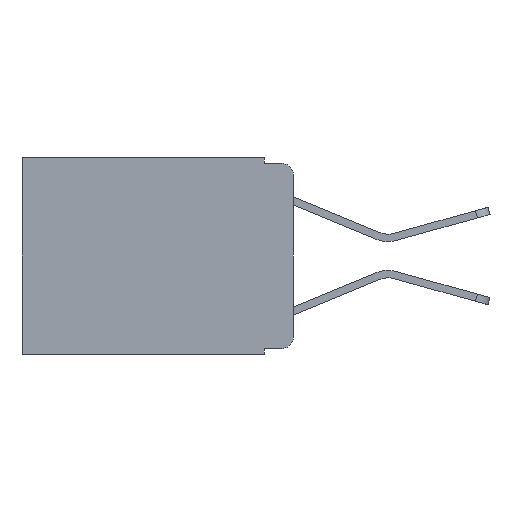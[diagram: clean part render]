
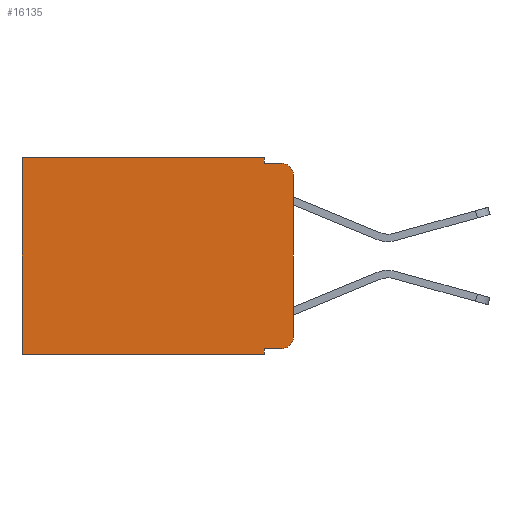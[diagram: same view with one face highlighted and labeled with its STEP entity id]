
A CAD part, left-side view. The second image highlights one B-rep face of the part: STEP entity #16135.
In plain terms, the highlighted planar face has unit normal (-1, 0, 0).
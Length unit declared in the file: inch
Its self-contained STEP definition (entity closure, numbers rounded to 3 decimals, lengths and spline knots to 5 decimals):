
#930 = DIRECTION ( 'NONE',  ( 0., 0., -1. ) ) ;
#975 = AXIS2_PLACEMENT_3D ( 'NONE', #14373, #9306, #9220 ) ;
#996 = EDGE_CURVE ( 'NONE', #8106, #8178, #16025, .T. ) ;
#1023 = CIRCLE ( 'NONE', #5226, 0.02 ) ;
#1413 = DIRECTION ( 'NONE',  ( 0., -1., 0. ) ) ;
#1445 = DIRECTION ( 'NONE',  ( 0., 0., -1. ) ) ;
#1476 = EDGE_CURVE ( 'NONE', #8192, #5066, #4135, .T. ) ;
#1765 = FACE_OUTER_BOUND ( 'NONE', #11702, .T. ) ;
#2794 = CARTESIAN_POINT ( 'NONE',  ( 0.298, 0.473, 0. ) ) ;
#2833 = AXIS2_PLACEMENT_3D ( 'NONE', #5784, #11110, #16434 ) ;
#2936 = ORIENTED_EDGE ( 'NONE', *, *, #5805, .F. ) ;
#3048 = CARTESIAN_POINT ( 'NONE',  ( 0.298, 0.051, -0.333 ) ) ;
#3153 = DIRECTION ( 'NONE',  ( -1., 0., 0. ) ) ;
#3159 = EDGE_CURVE ( 'NONE', #16995, #5421, #5808, .T. ) ;
#3177 = ORIENTED_EDGE ( 'NONE', *, *, #3159, .F. ) ;
#3296 = CARTESIAN_POINT ( 'NONE',  ( 0.298, 0., -0.313 ) ) ;
#3312 = LINE ( 'NONE', #7144, #11149 ) ;
#3498 = EDGE_CURVE ( 'NONE', #16995, #8106, #12305, .T. ) ;
#4135 = LINE ( 'NONE', #5103, #10213 ) ;
#4158 = CARTESIAN_POINT ( 'NONE',  ( 0.298, 0.473, 0. ) ) ;
#4216 = DIRECTION ( 'NONE',  ( 0., 0., -1. ) ) ;
#4322 = LINE ( 'NONE', #5625, #15662 ) ;
#4462 = CARTESIAN_POINT ( 'NONE',  ( 0.298, 0.02, -0.333 ) ) ;
#4895 = LINE ( 'NONE', #14287, #6115 ) ;
#5066 = VERTEX_POINT ( 'NONE', #14925 ) ;
#5103 = CARTESIAN_POINT ( 'NONE',  ( 0.298, 0.051, -0.01 ) ) ;
#5226 = AXIS2_PLACEMENT_3D ( 'NONE', #12319, #3153, #4216 ) ;
#5421 = VERTEX_POINT ( 'NONE', #7190 ) ;
#5423 = VERTEX_POINT ( 'NONE', #8684 ) ;
#5426 = CARTESIAN_POINT ( 'NONE',  ( 0.298, 0.051, -0.333 ) ) ;
#5625 = CARTESIAN_POINT ( 'NONE',  ( 0.298, 0., 0. ) ) ;
#5691 = LINE ( 'NONE', #11283, #7741 ) ;
#5784 = CARTESIAN_POINT ( 'NONE',  ( 0.298, 0., 0. ) ) ;
#5805 = EDGE_CURVE ( 'NONE', #5423, #8178, #4322, .T. ) ;
#5808 = LINE ( 'NONE', #7441, #16884 ) ;
#6003 = CARTESIAN_POINT ( 'NONE',  ( 0.298, 0.051, 0. ) ) ;
#6020 = ORIENTED_EDGE ( 'NONE', *, *, #8241, .T. ) ;
#6115 = VECTOR ( 'NONE', #930, 39.37008 ) ;
#6251 = EDGE_CURVE ( 'NONE', #5421, #10472, #3312, .T. ) ;
#6329 = EDGE_CURVE ( 'NONE', #16472, #9595, #5691, .T. ) ;
#6576 = VECTOR ( 'NONE', #1445, 39.37008 ) ;
#6862 = EDGE_CURVE ( 'NONE', #16472, #8192, #4895, .T. ) ;
#6928 = LINE ( 'NONE', #4158, #6576 ) ;
#7073 = PLANE ( 'NONE',  #2833 ) ;
#7144 = CARTESIAN_POINT ( 'NONE',  ( 0.298, 0., -0.343 ) ) ;
#7190 = CARTESIAN_POINT ( 'NONE',  ( 0.298, 0.051, -0.343 ) ) ;
#7256 = CARTESIAN_POINT ( 'NONE',  ( 0.298, 0.473, -0.343 ) ) ;
#7322 = ORIENTED_EDGE ( 'NONE', *, *, #1476, .F. ) ;
#7339 = ORIENTED_EDGE ( 'NONE', *, *, #996, .T. ) ;
#7441 = CARTESIAN_POINT ( 'NONE',  ( 0.298, 0.051, 0. ) ) ;
#7741 = VECTOR ( 'NONE', #9791, 39.37008 ) ;
#7961 = ORIENTED_EDGE ( 'NONE', *, *, #6862, .F. ) ;
#8087 = ORIENTED_EDGE ( 'NONE', *, *, #3498, .T. ) ;
#8106 = VERTEX_POINT ( 'NONE', #4462 ) ;
#8178 = VERTEX_POINT ( 'NONE', #3296 ) ;
#8192 = VERTEX_POINT ( 'NONE', #16401 ) ;
#8241 = EDGE_CURVE ( 'NONE', #9595, #10472, #6928, .T. ) ;
#8551 = ORIENTED_EDGE ( 'NONE', *, *, #12095, .T. ) ;
#8684 = CARTESIAN_POINT ( 'NONE',  ( 0.298, 0., -0.03 ) ) ;
#9220 = DIRECTION ( 'NONE',  ( 0., 0., -1. ) ) ;
#9306 = DIRECTION ( 'NONE',  ( -1., 0., 0. ) ) ;
#9310 = VECTOR ( 'NONE', #9506, 39.37008 ) ;
#9506 = DIRECTION ( 'NONE',  ( 0., -1., 0. ) ) ;
#9595 = VERTEX_POINT ( 'NONE', #2794 ) ;
#9791 = DIRECTION ( 'NONE',  ( 0., 1., 0. ) ) ;
#10213 = VECTOR ( 'NONE', #1413, 39.37008 ) ;
#10472 = VERTEX_POINT ( 'NONE', #7256 ) ;
#11110 = DIRECTION ( 'NONE',  ( 1., 0., 0. ) ) ;
#11149 = VECTOR ( 'NONE', #15015, 39.37008 ) ;
#11283 = CARTESIAN_POINT ( 'NONE',  ( 0.298, 0., 0. ) ) ;
#11702 = EDGE_LOOP ( 'NONE', ( #2936, #8551, #7322, #7961, #17272, #6020, #15754, #3177, #8087, #7339 ) ) ;
#12095 = EDGE_CURVE ( 'NONE', #5423, #5066, #1023, .T. ) ;
#12305 = LINE ( 'NONE', #3048, #9310 ) ;
#12319 = CARTESIAN_POINT ( 'NONE',  ( 0.298, 0.02, -0.03 ) ) ;
#13301 = DIRECTION ( 'NONE',  ( 0., 0., -1. ) ) ;
#14287 = CARTESIAN_POINT ( 'NONE',  ( 0.298, 0.051, 0. ) ) ;
#14373 = CARTESIAN_POINT ( 'NONE',  ( 0.298, 0.02, -0.313 ) ) ;
#14925 = CARTESIAN_POINT ( 'NONE',  ( 0.298, 0.02, -0.01 ) ) ;
#15015 = DIRECTION ( 'NONE',  ( 0., 1., 0. ) ) ;
#15662 = VECTOR ( 'NONE', #13301, 39.37008 ) ;
#15754 = ORIENTED_EDGE ( 'NONE', *, *, #6251, .F. ) ;
#16025 = CIRCLE ( 'NONE', #975, 0.02 ) ;
#16135 = ADVANCED_FACE ( 'NONE', ( #1765 ), #7073, .F. ) ;
#16401 = CARTESIAN_POINT ( 'NONE',  ( 0.298, 0.051, -0.01 ) ) ;
#16434 = DIRECTION ( 'NONE',  ( 0., 0., -1. ) ) ;
#16472 = VERTEX_POINT ( 'NONE', #6003 ) ;
#16718 = DIRECTION ( 'NONE',  ( 0., 0., -1. ) ) ;
#16884 = VECTOR ( 'NONE', #16718, 39.37008 ) ;
#16995 = VERTEX_POINT ( 'NONE', #5426 ) ;
#17272 = ORIENTED_EDGE ( 'NONE', *, *, #6329, .T. ) ;
